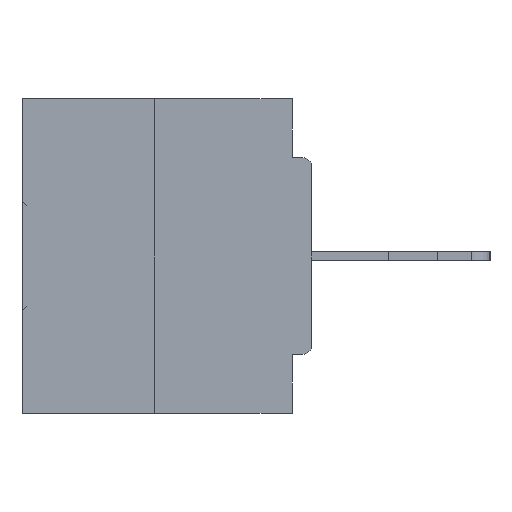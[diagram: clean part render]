
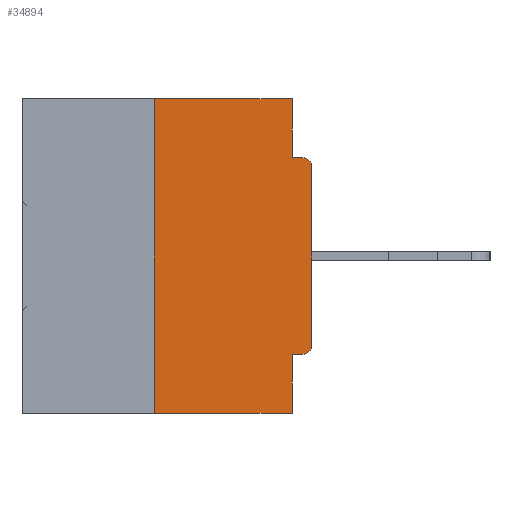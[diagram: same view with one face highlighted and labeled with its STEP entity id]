
A CAD part, left-side view. The second image highlights one B-rep face of the part: STEP entity #34894.
In plain terms, the highlighted planar face has unit normal (-1, 0, 0).
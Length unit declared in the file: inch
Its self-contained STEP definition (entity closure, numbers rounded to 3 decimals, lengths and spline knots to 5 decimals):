
#224 = CARTESIAN_POINT ( 'NONE',  ( 0., 0.25, -0.5 ) ) ;
#359 = VERTEX_POINT ( 'NONE', #38573 ) ;
#796 = EDGE_CURVE ( 'NONE', #5133, #26057, #23031, .T. ) ;
#1246 = VECTOR ( 'NONE', #1461, 39.37008 ) ;
#1461 = DIRECTION ( 'NONE',  ( 0., 0., -1. ) ) ;
#1725 = CARTESIAN_POINT ( 'NONE',  ( 0., 0.25, 0. ) ) ;
#1826 = LINE ( 'NONE', #32559, #36137 ) ;
#2090 = DIRECTION ( 'NONE',  ( -1., 0., 0. ) ) ;
#2927 = CARTESIAN_POINT ( 'NONE',  ( 0., 0.015, -0.0935 ) ) ;
#3243 = ORIENTED_EDGE ( 'NONE', *, *, #15251, .T. ) ;
#3347 = ORIENTED_EDGE ( 'NONE', *, *, #796, .F. ) ;
#3525 = CARTESIAN_POINT ( 'NONE',  ( 0., 0.015, -0.4065 ) ) ;
#4615 = CARTESIAN_POINT ( 'NONE',  ( 0., 0.031, -0.5 ) ) ;
#5133 = VERTEX_POINT ( 'NONE', #33997 ) ;
#5991 = EDGE_CURVE ( 'NONE', #17445, #29953, #27905, .T. ) ;
#6083 = PLANE ( 'NONE',  #24390 ) ;
#6199 = VECTOR ( 'NONE', #20524, 39.37008 ) ;
#6337 = LINE ( 'NONE', #24099, #37704 ) ;
#6683 = EDGE_CURVE ( 'NONE', #359, #33287, #17906, .T. ) ;
#7397 = VECTOR ( 'NONE', #22930, 39.37008 ) ;
#7416 = EDGE_CURVE ( 'NONE', #25995, #27695, #17347, .T. ) ;
#7763 = CARTESIAN_POINT ( 'NONE',  ( 0., 0., -0.3915 ) ) ;
#8236 = ORIENTED_EDGE ( 'NONE', *, *, #27096, .F. ) ;
#8929 = LINE ( 'NONE', #18427, #24763 ) ;
#9190 = DIRECTION ( 'NONE',  ( 1., 0., 0. ) ) ;
#11123 = ORIENTED_EDGE ( 'NONE', *, *, #6683, .F. ) ;
#12574 = EDGE_CURVE ( 'NONE', #27695, #17445, #8929, .T. ) ;
#13010 = CARTESIAN_POINT ( 'NONE',  ( 0., 0.015, -0.1085 ) ) ;
#15251 = EDGE_CURVE ( 'NONE', #23352, #33287, #37803, .T. ) ;
#15885 = ORIENTED_EDGE ( 'NONE', *, *, #7416, .T. ) ;
#16137 = DIRECTION ( 'NONE',  ( 0., 0., -1. ) ) ;
#17347 = CIRCLE ( 'NONE', #17944, 0.015 ) ;
#17445 = VERTEX_POINT ( 'NONE', #17980 ) ;
#17906 = LINE ( 'NONE', #4615, #1246 ) ;
#17944 = AXIS2_PLACEMENT_3D ( 'NONE', #20913, #2090, #24100 ) ;
#17980 = CARTESIAN_POINT ( 'NONE',  ( 0., 0., -0.1085 ) ) ;
#18120 = EDGE_LOOP ( 'NONE', ( #3347, #18356, #3243, #11123, #33999, #15885, #32608, #25599, #22075, #8236 ) ) ;
#18356 = ORIENTED_EDGE ( 'NONE', *, *, #24506, .F. ) ;
#18427 = CARTESIAN_POINT ( 'NONE',  ( 0., 0., 0. ) ) ;
#19424 = CARTESIAN_POINT ( 'NONE',  ( 0., 0.031, 0. ) ) ;
#19525 = CARTESIAN_POINT ( 'NONE',  ( 0., 0.031, -0.5 ) ) ;
#19681 = CARTESIAN_POINT ( 'NONE',  ( 0., 0.46, -0.5 ) ) ;
#20524 = DIRECTION ( 'NONE',  ( 0., 0., 1. ) ) ;
#20913 = CARTESIAN_POINT ( 'NONE',  ( 0., 0.015, -0.3915 ) ) ;
#20979 = CARTESIAN_POINT ( 'NONE',  ( 0., 0.46, 0. ) ) ;
#21297 = VECTOR ( 'NONE', #23102, 39.37008 ) ;
#21960 = AXIS2_PLACEMENT_3D ( 'NONE', #13010, #34997, #16137 ) ;
#22075 = ORIENTED_EDGE ( 'NONE', *, *, #30794, .F. ) ;
#22316 = LINE ( 'NONE', #29395, #21297 ) ;
#22420 = DIRECTION ( 'NONE',  ( 0., -1., 0. ) ) ;
#22930 = DIRECTION ( 'NONE',  ( 0., -1., 0. ) ) ;
#23031 = LINE ( 'NONE', #20979, #37609 ) ;
#23102 = DIRECTION ( 'NONE',  ( 0., -1., 0. ) ) ;
#23352 = VERTEX_POINT ( 'NONE', #224 ) ;
#23767 = EDGE_CURVE ( 'NONE', #25995, #359, #1826, .T. ) ;
#24098 = FACE_OUTER_BOUND ( 'NONE', #18120, .T. ) ;
#24099 = CARTESIAN_POINT ( 'NONE',  ( 0., 0.031, 0. ) ) ;
#24100 = DIRECTION ( 'NONE',  ( 0., 0., -1. ) ) ;
#24390 = AXIS2_PLACEMENT_3D ( 'NONE', #28146, #9190, #31291 ) ;
#24506 = EDGE_CURVE ( 'NONE', #23352, #5133, #30340, .T. ) ;
#24763 = VECTOR ( 'NONE', #34100, 39.37008 ) ;
#25599 = ORIENTED_EDGE ( 'NONE', *, *, #5991, .T. ) ;
#25995 = VERTEX_POINT ( 'NONE', #3525 ) ;
#26057 = VERTEX_POINT ( 'NONE', #19424 ) ;
#27096 = EDGE_CURVE ( 'NONE', #26057, #29995, #6337, .T. ) ;
#27256 = DIRECTION ( 'NONE',  ( 0., 0., -1. ) ) ;
#27695 = VERTEX_POINT ( 'NONE', #7763 ) ;
#27905 = CIRCLE ( 'NONE', #21960, 0.015 ) ;
#28146 = CARTESIAN_POINT ( 'NONE',  ( 0., 0.46, 0. ) ) ;
#29394 = DIRECTION ( 'NONE',  ( 0., 1., 0. ) ) ;
#29395 = CARTESIAN_POINT ( 'NONE',  ( 0., 0., -0.0935 ) ) ;
#29953 = VERTEX_POINT ( 'NONE', #2927 ) ;
#29995 = VERTEX_POINT ( 'NONE', #40473 ) ;
#30340 = LINE ( 'NONE', #1725, #6199 ) ;
#30794 = EDGE_CURVE ( 'NONE', #29995, #29953, #22316, .T. ) ;
#31291 = DIRECTION ( 'NONE',  ( 0., 0., -1. ) ) ;
#32559 = CARTESIAN_POINT ( 'NONE',  ( 0., 0., -0.4065 ) ) ;
#32608 = ORIENTED_EDGE ( 'NONE', *, *, #12574, .T. ) ;
#33287 = VERTEX_POINT ( 'NONE', #19525 ) ;
#33997 = CARTESIAN_POINT ( 'NONE',  ( 0., 0.25, 0. ) ) ;
#33999 = ORIENTED_EDGE ( 'NONE', *, *, #23767, .F. ) ;
#34100 = DIRECTION ( 'NONE',  ( 0., 0., 1. ) ) ;
#34894 = ADVANCED_FACE ( 'NONE', ( #24098 ), #6083, .F. ) ;
#34997 = DIRECTION ( 'NONE',  ( -1., 0., 0. ) ) ;
#36137 = VECTOR ( 'NONE', #29394, 39.37008 ) ;
#37609 = VECTOR ( 'NONE', #22420, 39.37008 ) ;
#37704 = VECTOR ( 'NONE', #27256, 39.37008 ) ;
#37803 = LINE ( 'NONE', #19681, #7397 ) ;
#38573 = CARTESIAN_POINT ( 'NONE',  ( 0., 0.031, -0.4065 ) ) ;
#40473 = CARTESIAN_POINT ( 'NONE',  ( 0., 0.031, -0.0935 ) ) ;
